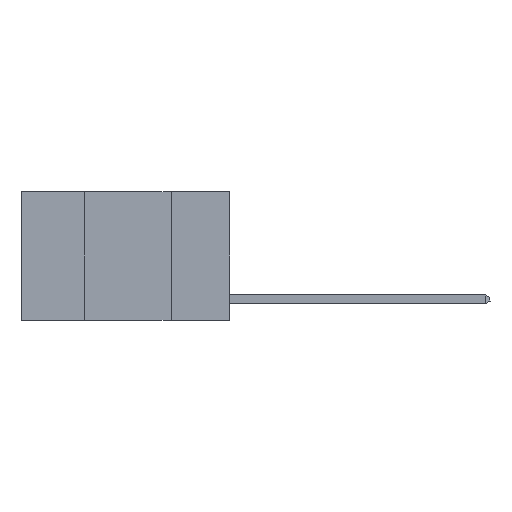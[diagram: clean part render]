
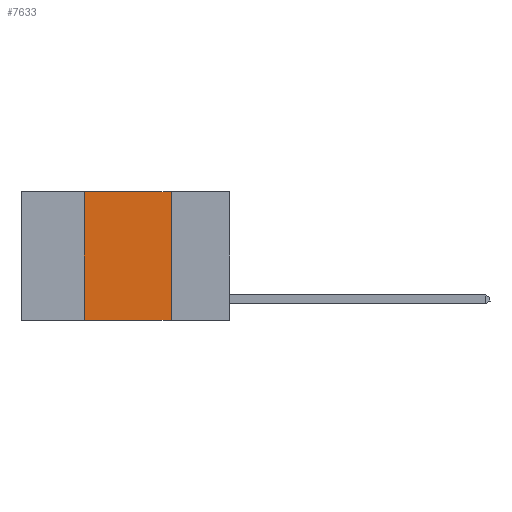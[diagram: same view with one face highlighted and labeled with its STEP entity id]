
A CAD part, left-side view. The second image highlights one B-rep face of the part: STEP entity #7633.
In plain terms, the highlighted planar face has unit normal (-1, 0, 0).
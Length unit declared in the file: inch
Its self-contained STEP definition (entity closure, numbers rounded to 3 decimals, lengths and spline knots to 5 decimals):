
#65 = VERTEX_POINT ( 'NONE', #8494 ) ;
#359 = EDGE_CURVE ( 'NONE', #8839, #12677, #14562, .T. ) ;
#727 = ORIENTED_EDGE ( 'NONE', *, *, #359, .F. ) ;
#959 = CARTESIAN_POINT ( 'NONE',  ( 0., 0.6, 0. ) ) ;
#1535 = CARTESIAN_POINT ( 'NONE',  ( 0., 0.42, 0. ) ) ;
#1960 = EDGE_CURVE ( 'NONE', #7912, #65, #7733, .T. ) ;
#2269 = DIRECTION ( 'NONE',  ( 1., 0., 0. ) ) ;
#3423 = FACE_OUTER_BOUND ( 'NONE', #7523, .T. ) ;
#3590 = CARTESIAN_POINT ( 'NONE',  ( 0., 0.42, 0. ) ) ;
#3902 = ORIENTED_EDGE ( 'NONE', *, *, #11056, .F. ) ;
#4597 = VECTOR ( 'NONE', #14938, 39.37008 ) ;
#4614 = CARTESIAN_POINT ( 'NONE',  ( 0., 0.6, 0. ) ) ;
#5250 = ORIENTED_EDGE ( 'NONE', *, *, #1960, .T. ) ;
#6172 = EDGE_CURVE ( 'NONE', #7912, #8839, #11490, .T. ) ;
#6328 = CARTESIAN_POINT ( 'NONE',  ( 0., 0.6, -0.37 ) ) ;
#6539 = DIRECTION ( 'NONE',  ( 0., 0., 1. ) ) ;
#7195 = PLANE ( 'NONE',  #14323 ) ;
#7328 = DIRECTION ( 'NONE',  ( 0., -1., 0. ) ) ;
#7523 = EDGE_LOOP ( 'NONE', ( #3902, #727, #12622, #5250 ) ) ;
#7633 = ADVANCED_FACE ( 'NONE', ( #3423 ), #7195, .F. ) ;
#7733 = LINE ( 'NONE', #6328, #9630 ) ;
#7912 = VERTEX_POINT ( 'NONE', #11791 ) ;
#8494 = CARTESIAN_POINT ( 'NONE',  ( 0., 0.17, -0.37 ) ) ;
#8531 = LINE ( 'NONE', #9924, #4597 ) ;
#8839 = VERTEX_POINT ( 'NONE', #3590 ) ;
#9630 = VECTOR ( 'NONE', #12747, 39.37008 ) ;
#9924 = CARTESIAN_POINT ( 'NONE',  ( 0., 0.17, 0. ) ) ;
#10988 = DIRECTION ( 'NONE',  ( 0., 0., -1. ) ) ;
#11056 = EDGE_CURVE ( 'NONE', #12677, #65, #8531, .T. ) ;
#11490 = LINE ( 'NONE', #1535, #11511 ) ;
#11511 = VECTOR ( 'NONE', #6539, 39.37008 ) ;
#11791 = CARTESIAN_POINT ( 'NONE',  ( 0., 0.42, -0.37 ) ) ;
#12440 = VECTOR ( 'NONE', #7328, 39.37008 ) ;
#12622 = ORIENTED_EDGE ( 'NONE', *, *, #6172, .F. ) ;
#12677 = VERTEX_POINT ( 'NONE', #12894 ) ;
#12747 = DIRECTION ( 'NONE',  ( 0., -1., 0. ) ) ;
#12894 = CARTESIAN_POINT ( 'NONE',  ( 0., 0.17, 0. ) ) ;
#14323 = AXIS2_PLACEMENT_3D ( 'NONE', #959, #2269, #10988 ) ;
#14562 = LINE ( 'NONE', #4614, #12440 ) ;
#14938 = DIRECTION ( 'NONE',  ( 0., 0., -1. ) ) ;
